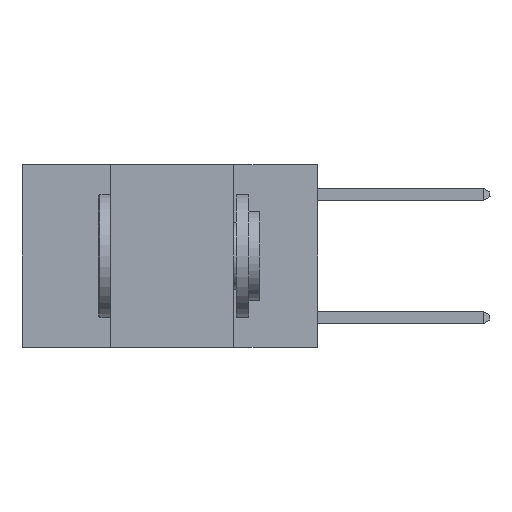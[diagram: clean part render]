
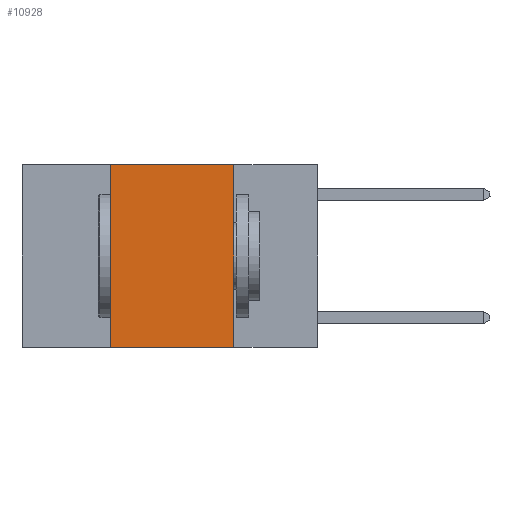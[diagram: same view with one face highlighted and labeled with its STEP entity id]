
A CAD part, left-side view. The second image highlights one B-rep face of the part: STEP entity #10928.
In plain terms, the highlighted planar face has unit normal (-1, 0, 0).
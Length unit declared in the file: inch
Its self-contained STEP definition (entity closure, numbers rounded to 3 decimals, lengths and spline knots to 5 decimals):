
#66 = CARTESIAN_POINT ( 'NONE',  ( 0., 0.17, -0.37 ) ) ;
#229 = CARTESIAN_POINT ( 'NONE',  ( 0., 0.17, 0. ) ) ;
#1043 = VERTEX_POINT ( 'NONE', #12816 ) ;
#1326 = DIRECTION ( 'NONE',  ( 0., 0., -1. ) ) ;
#1418 = VECTOR ( 'NONE', #6482, 39.37008 ) ;
#1477 = EDGE_CURVE ( 'NONE', #10704, #1043, #3842, .T. ) ;
#2223 = VECTOR ( 'NONE', #6908, 39.37008 ) ;
#2282 = EDGE_CURVE ( 'NONE', #1043, #10362, #6498, .T. ) ;
#2468 = VECTOR ( 'NONE', #11917, 39.37008 ) ;
#3485 = FACE_OUTER_BOUND ( 'NONE', #4189, .T. ) ;
#3683 = DIRECTION ( 'NONE',  ( 0., 0., -1. ) ) ;
#3842 = LINE ( 'NONE', #12852, #2468 ) ;
#4189 = EDGE_LOOP ( 'NONE', ( #5915, #5351, #10345, #12009 ) ) ;
#4692 = AXIS2_PLACEMENT_3D ( 'NONE', #7547, #7673, #3683 ) ;
#5185 = VERTEX_POINT ( 'NONE', #5538 ) ;
#5351 = ORIENTED_EDGE ( 'NONE', *, *, #1477, .F. ) ;
#5538 = CARTESIAN_POINT ( 'NONE',  ( 0., 0.42, -0.37 ) ) ;
#5915 = ORIENTED_EDGE ( 'NONE', *, *, #2282, .F. ) ;
#5917 = CARTESIAN_POINT ( 'NONE',  ( 0., 0.42, 0. ) ) ;
#5967 = EDGE_CURVE ( 'NONE', #5185, #10362, #6548, .T. ) ;
#6482 = DIRECTION ( 'NONE',  ( 0., -1., 0. ) ) ;
#6498 = LINE ( 'NONE', #229, #9037 ) ;
#6548 = LINE ( 'NONE', #12590, #1418 ) ;
#6908 = DIRECTION ( 'NONE',  ( 0., 0., 1. ) ) ;
#7547 = CARTESIAN_POINT ( 'NONE',  ( 0., 0.6, 0. ) ) ;
#7673 = DIRECTION ( 'NONE',  ( 1., 0., 0. ) ) ;
#7879 = LINE ( 'NONE', #5917, #2223 ) ;
#8094 = CARTESIAN_POINT ( 'NONE',  ( 0., 0.42, 0. ) ) ;
#9037 = VECTOR ( 'NONE', #1326, 39.37008 ) ;
#9260 = EDGE_CURVE ( 'NONE', #5185, #10704, #7879, .T. ) ;
#10345 = ORIENTED_EDGE ( 'NONE', *, *, #9260, .F. ) ;
#10362 = VERTEX_POINT ( 'NONE', #66 ) ;
#10704 = VERTEX_POINT ( 'NONE', #8094 ) ;
#10928 = ADVANCED_FACE ( 'NONE', ( #3485 ), #11830, .F. ) ;
#11830 = PLANE ( 'NONE',  #4692 ) ;
#11917 = DIRECTION ( 'NONE',  ( 0., -1., 0. ) ) ;
#12009 = ORIENTED_EDGE ( 'NONE', *, *, #5967, .T. ) ;
#12590 = CARTESIAN_POINT ( 'NONE',  ( 0., 0.6, -0.37 ) ) ;
#12816 = CARTESIAN_POINT ( 'NONE',  ( 0., 0.17, 0. ) ) ;
#12852 = CARTESIAN_POINT ( 'NONE',  ( 0., 0.6, 0. ) ) ;
